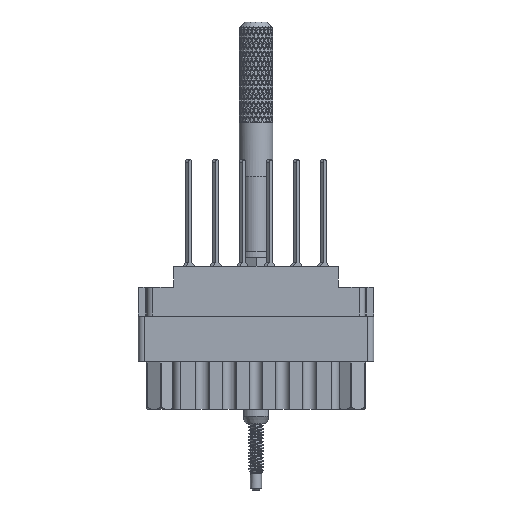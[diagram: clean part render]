
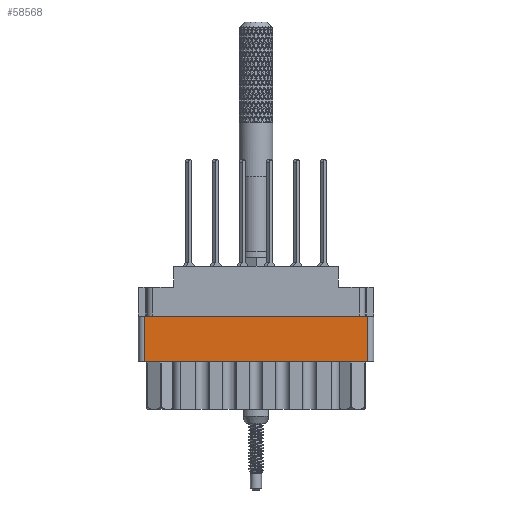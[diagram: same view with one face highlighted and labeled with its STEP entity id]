
A CAD part, front view. The second image highlights one B-rep face of the part: STEP entity #58568.
In plain terms, the highlighted planar face has unit normal (0, -1, 0).
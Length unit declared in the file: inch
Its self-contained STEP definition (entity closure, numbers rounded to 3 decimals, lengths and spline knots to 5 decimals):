
#6956 = LINE ( 'NONE', #125446, #94112 ) ;
#9549 = DIRECTION ( 'NONE',  ( 0., 0., 1. ) ) ;
#11140 = EDGE_CURVE ( 'NONE', #105435, #134523, #144084, .T. ) ;
#12046 = LINE ( 'NONE', #176118, #89261 ) ;
#21452 = CARTESIAN_POINT ( 'NONE',  ( 0.624, -0.343, -0.529 ) ) ;
#27621 = EDGE_CURVE ( 'NONE', #134523, #114451, #127077, .T. ) ;
#35271 = VECTOR ( 'NONE', #189702, 39.37008 ) ;
#53198 = EDGE_LOOP ( 'NONE', ( #87344, #168985, #181389, #84924 ) ) ;
#53579 = CARTESIAN_POINT ( 'NONE',  ( -0.624, -0.343, -0.798 ) ) ;
#58568 = ADVANCED_FACE ( 'NONE', ( #170091 ), #94410, .T. ) ;
#72273 = DIRECTION ( 'NONE',  ( 1., 0., 0. ) ) ;
#78175 = CARTESIAN_POINT ( 'NONE',  ( -0.624, -0.343, -0.529 ) ) ;
#84924 = ORIENTED_EDGE ( 'NONE', *, *, #162146, .F. ) ;
#87344 = ORIENTED_EDGE ( 'NONE', *, *, #27621, .F. ) ;
#89261 = VECTOR ( 'NONE', #72273, 39.37008 ) ;
#90152 = VECTOR ( 'NONE', #9549, 39.37008 ) ;
#94112 = VECTOR ( 'NONE', #184641, 39.37008 ) ;
#94410 = PLANE ( 'NONE',  #189921 ) ;
#105435 = VERTEX_POINT ( 'NONE', #21452 ) ;
#113778 = DIRECTION ( 'NONE',  ( 0., -1., 0. ) ) ;
#114451 = VERTEX_POINT ( 'NONE', #160208 ) ;
#124184 = CARTESIAN_POINT ( 'NONE',  ( -0.624, -0.343, -0.798 ) ) ;
#125446 = CARTESIAN_POINT ( 'NONE',  ( 0.624, -0.343, -0.798 ) ) ;
#127077 = LINE ( 'NONE', #124184, #90152 ) ;
#134523 = VERTEX_POINT ( 'NONE', #78175 ) ;
#140991 = DIRECTION ( 'NONE',  ( 0., 0., -1. ) ) ;
#144084 = LINE ( 'NONE', #188736, #35271 ) ;
#153701 = VERTEX_POINT ( 'NONE', #174789 ) ;
#160208 = CARTESIAN_POINT ( 'NONE',  ( -0.624, -0.343, -0.277 ) ) ;
#162146 = EDGE_CURVE ( 'NONE', #114451, #153701, #12046, .T. ) ;
#168985 = ORIENTED_EDGE ( 'NONE', *, *, #11140, .F. ) ;
#170091 = FACE_OUTER_BOUND ( 'NONE', #53198, .T. ) ;
#174789 = CARTESIAN_POINT ( 'NONE',  ( 0.624, -0.343, -0.277 ) ) ;
#176118 = CARTESIAN_POINT ( 'NONE',  ( -0.656, -0.343, -0.277 ) ) ;
#181389 = ORIENTED_EDGE ( 'NONE', *, *, #183715, .T. ) ;
#183715 = EDGE_CURVE ( 'NONE', #105435, #153701, #6956, .T. ) ;
#184641 = DIRECTION ( 'NONE',  ( 0., 0., 1. ) ) ;
#188736 = CARTESIAN_POINT ( 'NONE',  ( 0.624, -0.343, -0.529 ) ) ;
#189702 = DIRECTION ( 'NONE',  ( -1., 0., 0. ) ) ;
#189921 = AXIS2_PLACEMENT_3D ( 'NONE', #53579, #113778, #140991 ) ;
